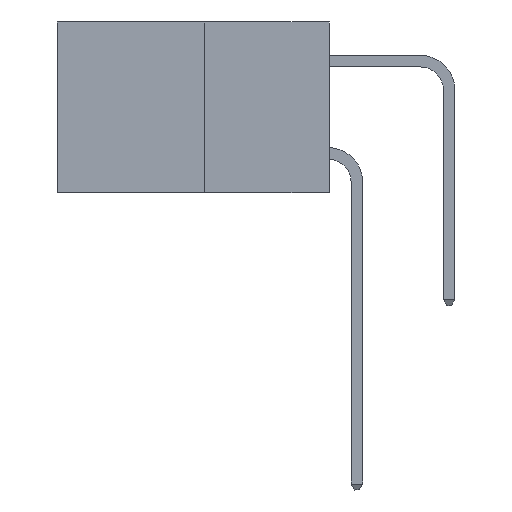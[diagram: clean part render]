
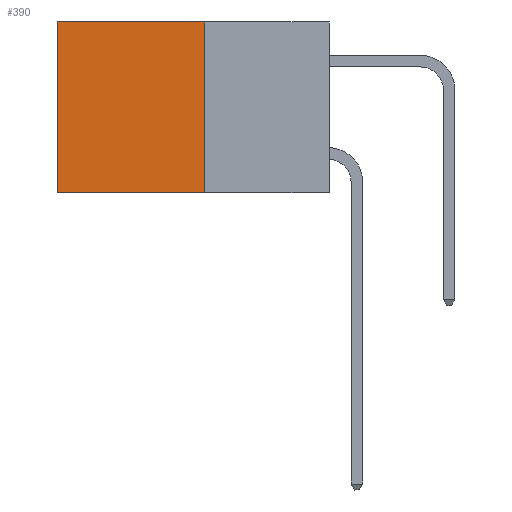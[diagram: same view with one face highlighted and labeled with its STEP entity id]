
A CAD part, left-side view. The second image highlights one B-rep face of the part: STEP entity #390.
In plain terms, the highlighted planar face has unit normal (-1, 0, 0).
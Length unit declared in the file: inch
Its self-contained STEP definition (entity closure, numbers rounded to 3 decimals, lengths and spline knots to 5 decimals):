
#106 = CARTESIAN_POINT ( 'NONE',  ( 0.277, 0.27, -0.37 ) ) ;
#145 = ORIENTED_EDGE ( 'NONE', *, *, #245, .F. ) ;
#245 = EDGE_CURVE ( 'NONE', #8520, #8220, #9099, .T. ) ;
#390 = ADVANCED_FACE ( 'NONE', ( #9508 ), #5851, .F. ) ;
#417 = CARTESIAN_POINT ( 'NONE',  ( 0.277, 0.27, 0. ) ) ;
#521 = ORIENTED_EDGE ( 'NONE', *, *, #4317, .F. ) ;
#1538 = ORIENTED_EDGE ( 'NONE', *, *, #6827, .T. ) ;
#2237 = CARTESIAN_POINT ( 'NONE',  ( 0.277, 0.59, -0.37 ) ) ;
#2272 = DIRECTION ( 'NONE',  ( 1., 0., 0. ) ) ;
#2414 = EDGE_CURVE ( 'NONE', #8520, #3618, #10291, .T. ) ;
#2850 = DIRECTION ( 'NONE',  ( 0., 1., 0. ) ) ;
#2968 = CARTESIAN_POINT ( 'NONE',  ( 0.277, 0.27, 0. ) ) ;
#3387 = DIRECTION ( 'NONE',  ( 0., 0., -1. ) ) ;
#3618 = VERTEX_POINT ( 'NONE', #6580 ) ;
#3972 = DIRECTION ( 'NONE',  ( 0., 0., -1. ) ) ;
#4317 = EDGE_CURVE ( 'NONE', #8220, #10430, #9996, .T. ) ;
#4409 = VECTOR ( 'NONE', #5887, 39.37008 ) ;
#5271 = CARTESIAN_POINT ( 'NONE',  ( 0.277, 0.27, -0.37 ) ) ;
#5851 = PLANE ( 'NONE',  #9157 ) ;
#5879 = CARTESIAN_POINT ( 'NONE',  ( 0.277, 0.27, -0.37 ) ) ;
#5887 = DIRECTION ( 'NONE',  ( 0., 1., 0. ) ) ;
#6118 = EDGE_LOOP ( 'NONE', ( #1538, #521, #145, #7639 ) ) ;
#6131 = CARTESIAN_POINT ( 'NONE',  ( 0.277, 0.27, -0.37 ) ) ;
#6339 = VECTOR ( 'NONE', #9050, 39.37008 ) ;
#6580 = CARTESIAN_POINT ( 'NONE',  ( 0.277, 0.59, 0. ) ) ;
#6827 = EDGE_CURVE ( 'NONE', #3618, #10430, #6874, .T. ) ;
#6874 = LINE ( 'NONE', #2237, #6339 ) ;
#7639 = ORIENTED_EDGE ( 'NONE', *, *, #2414, .T. ) ;
#8035 = VECTOR ( 'NONE', #2850, 39.37008 ) ;
#8220 = VERTEX_POINT ( 'NONE', #5879 ) ;
#8520 = VERTEX_POINT ( 'NONE', #417 ) ;
#8534 = CARTESIAN_POINT ( 'NONE',  ( 0.277, 0.59, -0.37 ) ) ;
#8841 = VECTOR ( 'NONE', #3387, 39.37008 ) ;
#9050 = DIRECTION ( 'NONE',  ( 0., 0., -1. ) ) ;
#9099 = LINE ( 'NONE', #106, #8841 ) ;
#9157 = AXIS2_PLACEMENT_3D ( 'NONE', #5271, #2272, #3972 ) ;
#9508 = FACE_OUTER_BOUND ( 'NONE', #6118, .T. ) ;
#9996 = LINE ( 'NONE', #6131, #4409 ) ;
#10291 = LINE ( 'NONE', #2968, #8035 ) ;
#10430 = VERTEX_POINT ( 'NONE', #8534 ) ;
